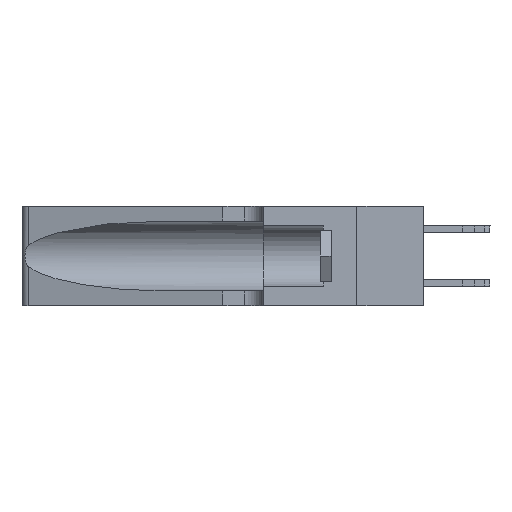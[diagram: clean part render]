
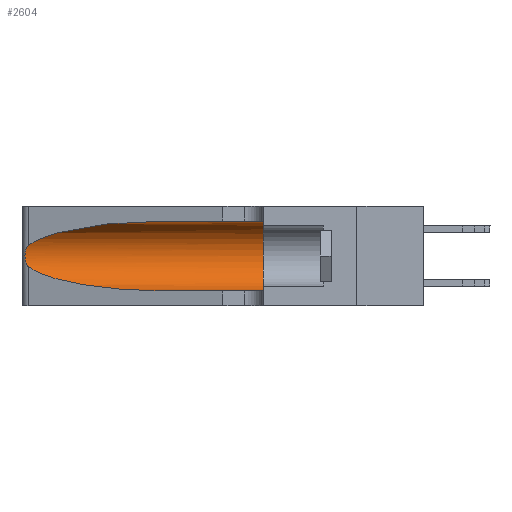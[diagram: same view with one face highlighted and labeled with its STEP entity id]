
A CAD part, left-side view. The second image highlights one B-rep face of the part: STEP entity #2604.
In plain terms, the highlighted cylindrical face has radius 3.308 mm (diameter 6.617 mm), a partial arc.
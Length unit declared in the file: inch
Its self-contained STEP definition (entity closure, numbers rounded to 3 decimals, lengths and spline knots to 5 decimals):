
#269 = CARTESIAN_POINT ( 'NONE',  ( 0.1305, 1.61858, 0.31525 ) ) ;
#329 = CARTESIAN_POINT ( 'NONE',  ( 0.1305, 0.35, 0.185 ) ) ;
#706 = ORIENTED_EDGE ( 'NONE', *, *, #10111, .T. ) ;
#1078 = CARTESIAN_POINT ( 'NONE',  ( 0.25787, 1.23484, 0.2124 ) ) ;
#1245 = CARTESIAN_POINT ( 'NONE',  ( 0.26075, 1.23896, 0.19203 ) ) ;
#1317 =( BOUNDED_CURVE ( )  B_SPLINE_CURVE ( 3, ( #8293, #13797, #21604, #23231 ),
 .UNSPECIFIED., .F., .T. ) 
 B_SPLINE_CURVE_WITH_KNOTS ( ( 4, 4 ),
 ( 1.5708, 2.84003 ),
 .UNSPECIFIED. ) 
 CURVE ( )  GEOMETRIC_REPRESENTATION_ITEM ( )  RATIONAL_B_SPLINE_CURVE ( ( 1., 0.87, 0.87, 1. ) ) 
 REPRESENTATION_ITEM ( '' )  );
#1471 = CARTESIAN_POINT ( 'NONE',  ( 0.1305, 0.35, 0.05475 ) ) ;
#1556 = VERTEX_POINT ( 'NONE', #3098 ) ;
#1677 = CARTESIAN_POINT ( 'NONE',  ( 0.25487, 1.22718, 0.14631 ) ) ;
#2604 = ADVANCED_FACE ( 'NONE', ( #3089 ), #5767, .F. ) ;
#3089 = FACE_OUTER_BOUND ( 'NONE', #12452, .T. ) ;
#3098 = CARTESIAN_POINT ( 'NONE',  ( 0.25487, 1.22718, 0.22369 ) ) ;
#3187 = CARTESIAN_POINT ( 'NONE',  ( 0.25639, 1.23186, 0.15144 ) ) ;
#4141 = VERTEX_POINT ( 'NONE', #18225 ) ;
#4423 = DIRECTION ( 'NONE',  ( 0., 0., 1. ) ) ;
#4450 = EDGE_CURVE ( 'NONE', #6088, #9383, #11030, .T. ) ;
#5129 = CARTESIAN_POINT ( 'NONE',  ( 0.1305, 0.72297, 0.05475 ) ) ;
#5767 = CYLINDRICAL_SURFACE ( 'NONE', #16736, 0.13025 ) ;
#6065 = CARTESIAN_POINT ( 'NONE',  ( 0.25487, 1.22718, 0.14631 ) ) ;
#6088 = VERTEX_POINT ( 'NONE', #22989 ) ;
#6746 = VERTEX_POINT ( 'NONE', #1677 ) ;
#6783 = CARTESIAN_POINT ( 'NONE',  ( 0.25854, 1.2359, 0.20912 ) ) ;
#7035 = CARTESIAN_POINT ( 'NONE',  ( 0.25487, 1.22718, 0.22369 ) ) ;
#7089 = VECTOR ( 'NONE', #15471, 39.37008 ) ;
#7943 = CARTESIAN_POINT ( 'NONE',  ( 0.1305, 0.72297, 0.05475 ) ) ;
#8293 = CARTESIAN_POINT ( 'NONE',  ( 0.1305, 0.72297, 0.31525 ) ) ;
#9383 = VERTEX_POINT ( 'NONE', #1471 ) ;
#9605 = VERTEX_POINT ( 'NONE', #5129 ) ;
#9938 = ORIENTED_EDGE ( 'NONE', *, *, #22310, .T. ) ;
#10111 = EDGE_CURVE ( 'NONE', #1556, #6746, #11224, .T. ) ;
#10526 = CARTESIAN_POINT ( 'NONE',  ( 0.25789, 1.23486, 0.15765 ) ) ;
#11030 = CIRCLE ( 'NONE', #18525, 0.13025 ) ;
#11154 = DIRECTION ( 'NONE',  ( 0., -1., 0. ) ) ;
#11224 = B_SPLINE_CURVE_WITH_KNOTS ( 'NONE', 3,
 ( #7035, #20274, #18345, #1078, #6783, #16508, #1245, #20100, #18429, #14519, #10526, #3187, #22024, #21847 ),
 .UNSPECIFIED., .F., .F.,
 ( 4, 2, 2, 2, 2, 2, 4 ),
 ( 0., 0.00027, 0.00053, 0.00107, 0.0016, 0.00187, 0.00214 ),
 .UNSPECIFIED. ) ;
#11327 = DIRECTION ( 'NONE',  ( 0., -1., 0. ) ) ;
#11465 = CARTESIAN_POINT ( 'NONE',  ( 0.2373, 1.15595, 0.08982 ) ) ;
#12452 = EDGE_LOOP ( 'NONE', ( #16732, #706, #9938, #15906, #16084, #13653 ) ) ;
#13485 = DIRECTION ( 'NONE',  ( 0., 0., -1. ) ) ;
#13653 = ORIENTED_EDGE ( 'NONE', *, *, #17928, .F. ) ;
#13797 = CARTESIAN_POINT ( 'NONE',  ( 0.18966, 0.96281, 0.31525 ) ) ;
#14018 = EDGE_CURVE ( 'NONE', #9605, #9383, #18834, .T. ) ;
#14519 = CARTESIAN_POINT ( 'NONE',  ( 0.25856, 1.23593, 0.16098 ) ) ;
#15471 = DIRECTION ( 'NONE',  ( 0., -1., 0. ) ) ;
#15524 = DIRECTION ( 'NONE',  ( 0., 1., 0. ) ) ;
#15906 = ORIENTED_EDGE ( 'NONE', *, *, #14018, .T. ) ;
#16084 = ORIENTED_EDGE ( 'NONE', *, *, #4450, .F. ) ;
#16508 = CARTESIAN_POINT ( 'NONE',  ( 0.26018, 1.23835, 0.19895 ) ) ;
#16732 = ORIENTED_EDGE ( 'NONE', *, *, #21788, .T. ) ;
#16736 = AXIS2_PLACEMENT_3D ( 'NONE', #22561, #11154, #13485 ) ;
#17144 =( BOUNDED_CURVE ( )  B_SPLINE_CURVE ( 3, ( #6065, #11465, #19351, #7943 ),
 .UNSPECIFIED., .F., .F. ) 
 B_SPLINE_CURVE_WITH_KNOTS ( ( 4, 4 ),
 ( 3.44316, 4.71239 ),
 .UNSPECIFIED. ) 
 CURVE ( )  GEOMETRIC_REPRESENTATION_ITEM ( )  RATIONAL_B_SPLINE_CURVE ( ( 1., 0.87, 0.87, 1. ) ) 
 REPRESENTATION_ITEM ( '' )  );
#17928 = EDGE_CURVE ( 'NONE', #4141, #6088, #19594, .T. ) ;
#18225 = CARTESIAN_POINT ( 'NONE',  ( 0.1305, 0.72297, 0.31525 ) ) ;
#18345 = CARTESIAN_POINT ( 'NONE',  ( 0.25639, 1.23184, 0.21858 ) ) ;
#18429 = CARTESIAN_POINT ( 'NONE',  ( 0.26017, 1.23833, 0.17102 ) ) ;
#18525 = AXIS2_PLACEMENT_3D ( 'NONE', #329, #15524, #4423 ) ;
#18834 = LINE ( 'NONE', #20911, #24498 ) ;
#19351 = CARTESIAN_POINT ( 'NONE',  ( 0.18966, 0.96281, 0.05475 ) ) ;
#19594 = LINE ( 'NONE', #269, #7089 ) ;
#20100 = CARTESIAN_POINT ( 'NONE',  ( 0.26075, 1.23896, 0.178 ) ) ;
#20274 = CARTESIAN_POINT ( 'NONE',  ( 0.25555, 1.22994, 0.2215 ) ) ;
#20911 = CARTESIAN_POINT ( 'NONE',  ( 0.1305, 1.61858, 0.05475 ) ) ;
#21604 = CARTESIAN_POINT ( 'NONE',  ( 0.2373, 1.15595, 0.28018 ) ) ;
#21788 = EDGE_CURVE ( 'NONE', #4141, #1556, #1317, .T. ) ;
#21847 = CARTESIAN_POINT ( 'NONE',  ( 0.25487, 1.22718, 0.14631 ) ) ;
#22024 = CARTESIAN_POINT ( 'NONE',  ( 0.25555, 1.22993, 0.14849 ) ) ;
#22310 = EDGE_CURVE ( 'NONE', #6746, #9605, #17144, .T. ) ;
#22561 = CARTESIAN_POINT ( 'NONE',  ( 0.1305, 1.61858, 0.185 ) ) ;
#22989 = CARTESIAN_POINT ( 'NONE',  ( 0.1305, 0.35, 0.31525 ) ) ;
#23231 = CARTESIAN_POINT ( 'NONE',  ( 0.25487, 1.22718, 0.22369 ) ) ;
#24498 = VECTOR ( 'NONE', #11327, 39.37008 ) ;
